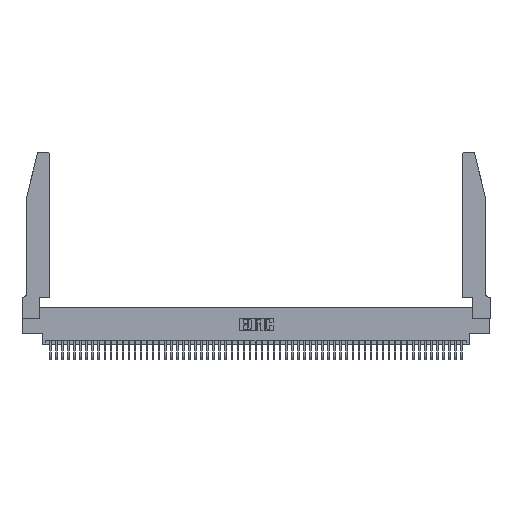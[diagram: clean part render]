
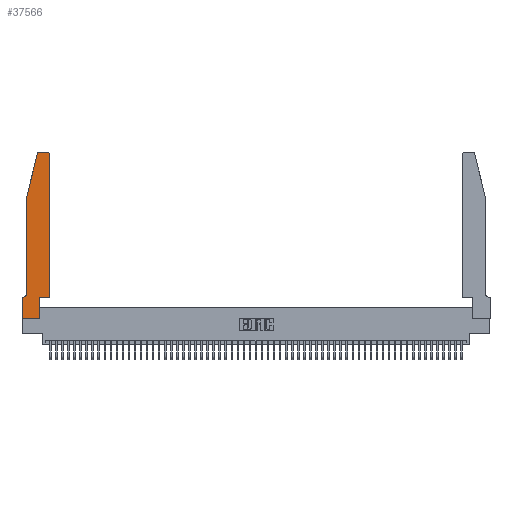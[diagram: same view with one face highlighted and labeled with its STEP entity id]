
A CAD part, top view. The second image highlights one B-rep face of the part: STEP entity #37566.
In plain terms, the highlighted planar face has unit normal (0, 0, 1).
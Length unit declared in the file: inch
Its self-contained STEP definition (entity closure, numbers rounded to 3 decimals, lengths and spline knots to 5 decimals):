
#264 = DIRECTION ( 'NONE',  ( 1., 0., 0. ) ) ;
#850 = CARTESIAN_POINT ( 'NONE',  ( 0.0055, 0.42, 0.37 ) ) ;
#1144 = VECTOR ( 'NONE', #38736, 39.37008 ) ;
#1408 = LINE ( 'NONE', #19178, #43872 ) ;
#2450 = DIRECTION ( 'NONE',  ( 0., 1., 0. ) ) ;
#4119 = EDGE_CURVE ( 'NONE', #5772, #39839, #33947, .T. ) ;
#4332 = CARTESIAN_POINT ( 'NONE',  ( 0.0755, 0.42, 0.37 ) ) ;
#5021 = DIRECTION ( 'NONE',  ( -1., 0., 0. ) ) ;
#5772 = VERTEX_POINT ( 'NONE', #14798 ) ;
#6760 = ORIENTED_EDGE ( 'NONE', *, *, #22245, .T. ) ;
#7665 = CARTESIAN_POINT ( 'NONE',  ( 0.0755, 2., 0.37 ) ) ;
#9285 = ORIENTED_EDGE ( 'NONE', *, *, #42238, .T. ) ;
#9904 = ORIENTED_EDGE ( 'NONE', *, *, #34793, .T. ) ;
#9963 = ORIENTED_EDGE ( 'NONE', *, *, #12445, .T. ) ;
#10392 = CARTESIAN_POINT ( 'NONE',  ( 0., 0.35, 0.37 ) ) ;
#11529 = LINE ( 'NONE', #48398, #33374 ) ;
#11602 = EDGE_CURVE ( 'NONE', #12504, #38790, #53228, .T. ) ;
#12072 = CARTESIAN_POINT ( 'NONE',  ( 0., 0., 0.37 ) ) ;
#12148 = CARTESIAN_POINT ( 'NONE',  ( 0.284, 2.75, 0.37 ) ) ;
#12408 = LINE ( 'NONE', #40321, #45134 ) ;
#12445 = EDGE_CURVE ( 'NONE', #14115, #22242, #11529, .T. ) ;
#12504 = VERTEX_POINT ( 'NONE', #7665 ) ;
#13017 = VECTOR ( 'NONE', #40576, 39.37008 ) ;
#13270 = CARTESIAN_POINT ( 'NONE',  ( 0.2865, 0., 0.37 ) ) ;
#13363 = VECTOR ( 'NONE', #2450, 39.37008 ) ;
#14115 = VERTEX_POINT ( 'NONE', #10392 ) ;
#14160 = CARTESIAN_POINT ( 'NONE',  ( 0.2605, 2.75, 0.37 ) ) ;
#14798 = CARTESIAN_POINT ( 'NONE',  ( 0.4505, 2.72, 0.37 ) ) ;
#15087 = ORIENTED_EDGE ( 'NONE', *, *, #44454, .T. ) ;
#15309 = CARTESIAN_POINT ( 'NONE',  ( 0.0755, 2., 0.37 ) ) ;
#15889 = EDGE_CURVE ( 'NONE', #22242, #33195, #20107, .T. ) ;
#16211 = DIRECTION ( 'NONE',  ( 0., 0., 1. ) ) ;
#16509 = DIRECTION ( 'NONE',  ( 0., 1., 0. ) ) ;
#16629 = AXIS2_PLACEMENT_3D ( 'NONE', #17119, #21249, #49894 ) ;
#16803 = VERTEX_POINT ( 'NONE', #18457 ) ;
#17119 = CARTESIAN_POINT ( 'NONE',  ( 0., 0.35, 0.37 ) ) ;
#18457 = CARTESIAN_POINT ( 'NONE',  ( 0.4505, 0.35, 0.37 ) ) ;
#18986 = VERTEX_POINT ( 'NONE', #45917 ) ;
#19039 = AXIS2_PLACEMENT_3D ( 'NONE', #40740, #16211, #44870 ) ;
#19178 = CARTESIAN_POINT ( 'NONE',  ( 0.4505, 0.35, 0.37 ) ) ;
#19756 = DIRECTION ( 'NONE',  ( 0., -1., 0. ) ) ;
#20107 = LINE ( 'NONE', #12072, #13017 ) ;
#20304 = ORIENTED_EDGE ( 'NONE', *, *, #33295, .T. ) ;
#21249 = DIRECTION ( 'NONE',  ( 0., 0., 1. ) ) ;
#22242 = VERTEX_POINT ( 'NONE', #45224 ) ;
#22245 = EDGE_CURVE ( 'NONE', #51839, #18986, #25956, .T. ) ;
#22689 = VECTOR ( 'NONE', #34529, 39.37008 ) ;
#23002 = CARTESIAN_POINT ( 'NONE',  ( 0.4505, 0.35, 0.37 ) ) ;
#24876 = VECTOR ( 'NONE', #16509, 39.37008 ) ;
#24976 = DIRECTION ( 'NONE',  ( 0., 0., 1. ) ) ;
#25956 = CIRCLE ( 'NONE', #51491, 0.03 ) ;
#25989 = ORIENTED_EDGE ( 'NONE', *, *, #50709, .T. ) ;
#27139 = VERTEX_POINT ( 'NONE', #49397 ) ;
#28225 = EDGE_CURVE ( 'NONE', #18986, #12504, #12408, .T. ) ;
#29677 = DIRECTION ( 'NONE',  ( 0., 0., -1. ) ) ;
#31164 = ORIENTED_EDGE ( 'NONE', *, *, #11602, .T. ) ;
#31614 = CARTESIAN_POINT ( 'NONE',  ( 0.4205, 2.75, 0.37 ) ) ;
#32739 = LINE ( 'NONE', #14160, #1144 ) ;
#33195 = VERTEX_POINT ( 'NONE', #13270 ) ;
#33295 = EDGE_CURVE ( 'NONE', #39839, #51839, #32739, .T. ) ;
#33374 = VECTOR ( 'NONE', #19756, 39.37008 ) ;
#33947 = CIRCLE ( 'NONE', #19039, 0.03 ) ;
#34526 = LINE ( 'NONE', #45161, #24876 ) ;
#34529 = DIRECTION ( 'NONE',  ( -1., 0., 0. ) ) ;
#34655 = VERTEX_POINT ( 'NONE', #47733 ) ;
#34793 = EDGE_CURVE ( 'NONE', #16803, #5772, #47382, .T. ) ;
#35854 = FACE_OUTER_BOUND ( 'NONE', #41616, .T. ) ;
#37514 = ORIENTED_EDGE ( 'NONE', *, *, #4119, .T. ) ;
#37566 = ADVANCED_FACE ( 'NONE', ( #35854 ), #45775, .T. ) ;
#38283 = AXIS2_PLACEMENT_3D ( 'NONE', #850, #29677, #5021 ) ;
#38623 = CARTESIAN_POINT ( 'NONE',  ( 0.0755, 0.35, 0.37 ) ) ;
#38736 = DIRECTION ( 'NONE',  ( -1., 0., 0. ) ) ;
#38790 = VERTEX_POINT ( 'NONE', #4332 ) ;
#39839 = VERTEX_POINT ( 'NONE', #31614 ) ;
#40321 = CARTESIAN_POINT ( 'NONE',  ( 0.0755, 2., 0.37 ) ) ;
#40576 = DIRECTION ( 'NONE',  ( 1., 0., 0. ) ) ;
#40740 = CARTESIAN_POINT ( 'NONE',  ( 0.4205, 2.72, 0.37 ) ) ;
#41616 = EDGE_LOOP ( 'NONE', ( #20304, #6760, #49725, #31164, #25989, #47129, #9963, #44616, #9285, #15087, #9904, #37514 ) ) ;
#42238 = EDGE_CURVE ( 'NONE', #33195, #27139, #34526, .T. ) ;
#43720 = DIRECTION ( 'NONE',  ( 1., 0., 0. ) ) ;
#43872 = VECTOR ( 'NONE', #43720, 39.37008 ) ;
#44454 = EDGE_CURVE ( 'NONE', #27139, #16803, #1408, .T. ) ;
#44616 = ORIENTED_EDGE ( 'NONE', *, *, #15889, .T. ) ;
#44870 = DIRECTION ( 'NONE',  ( 1., 0., 0. ) ) ;
#45134 = VECTOR ( 'NONE', #48386, 39.37008 ) ;
#45161 = CARTESIAN_POINT ( 'NONE',  ( 0.2865, 0.35, 0.37 ) ) ;
#45224 = CARTESIAN_POINT ( 'NONE',  ( 0., 0., 0.37 ) ) ;
#45775 = PLANE ( 'NONE',  #16629 ) ;
#45917 = CARTESIAN_POINT ( 'NONE',  ( 0.25487, 2.72718, 0.37 ) ) ;
#47129 = ORIENTED_EDGE ( 'NONE', *, *, #50819, .T. ) ;
#47382 = LINE ( 'NONE', #23002, #13363 ) ;
#47733 = CARTESIAN_POINT ( 'NONE',  ( 0.0055, 0.35, 0.37 ) ) ;
#48386 = DIRECTION ( 'NONE',  ( -0.239, -0.971, 0. ) ) ;
#48398 = CARTESIAN_POINT ( 'NONE',  ( 0., 0., 0.37 ) ) ;
#49397 = CARTESIAN_POINT ( 'NONE',  ( 0.2865, 0.35, 0.37 ) ) ;
#49510 = CARTESIAN_POINT ( 'NONE',  ( 0.284, 2.72, 0.37 ) ) ;
#49605 = CIRCLE ( 'NONE', #38283, 0.07 ) ;
#49725 = ORIENTED_EDGE ( 'NONE', *, *, #28225, .T. ) ;
#49894 = DIRECTION ( 'NONE',  ( 1., 0., 0. ) ) ;
#50709 = EDGE_CURVE ( 'NONE', #38790, #34655, #49605, .T. ) ;
#50819 = EDGE_CURVE ( 'NONE', #34655, #14115, #52803, .T. ) ;
#51491 = AXIS2_PLACEMENT_3D ( 'NONE', #49510, #24976, #264 ) ;
#51839 = VERTEX_POINT ( 'NONE', #12148 ) ;
#51958 = VECTOR ( 'NONE', #52212, 39.37008 ) ;
#52212 = DIRECTION ( 'NONE',  ( 0., -1., 0. ) ) ;
#52803 = LINE ( 'NONE', #38623, #22689 ) ;
#53228 = LINE ( 'NONE', #15309, #51958 ) ;
